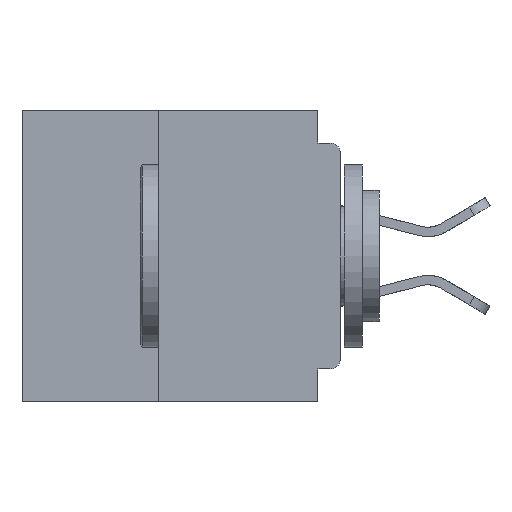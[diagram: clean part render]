
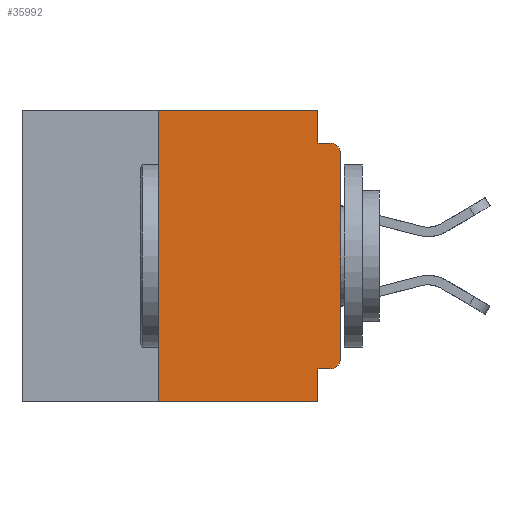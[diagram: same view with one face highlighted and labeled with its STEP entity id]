
A CAD part, left-side view. The second image highlights one B-rep face of the part: STEP entity #35992.
In plain terms, the highlighted planar face has unit normal (-1, 0, 0).
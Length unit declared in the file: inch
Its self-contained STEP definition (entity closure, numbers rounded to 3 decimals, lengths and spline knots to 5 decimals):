
#248 = VECTOR ( 'NONE', #33998, 39.37008 ) ;
#318 = VERTEX_POINT ( 'NONE', #36417 ) ;
#657 = CARTESIAN_POINT ( 'NONE',  ( 0., 0.031, -0.4 ) ) ;
#1243 = CARTESIAN_POINT ( 'NONE',  ( 0., 0.437, -0.4 ) ) ;
#1575 = CARTESIAN_POINT ( 'NONE',  ( 0., 0.015, -0.355 ) ) ;
#1850 = ORIENTED_EDGE ( 'NONE', *, *, #8075, .T. ) ;
#1880 = CARTESIAN_POINT ( 'NONE',  ( 0., 0.031, 0. ) ) ;
#3118 = VECTOR ( 'NONE', #18777, 39.37008 ) ;
#3287 = VECTOR ( 'NONE', #11905, 39.37008 ) ;
#3427 = VECTOR ( 'NONE', #29577, 39.37008 ) ;
#3503 = ORIENTED_EDGE ( 'NONE', *, *, #30465, .F. ) ;
#3931 = ORIENTED_EDGE ( 'NONE', *, *, #5375, .F. ) ;
#5300 = DIRECTION ( 'NONE',  ( 0., 0., -1. ) ) ;
#5311 = DIRECTION ( 'NONE',  ( -1., 0., 0. ) ) ;
#5351 = CARTESIAN_POINT ( 'NONE',  ( 0., 0.015, -0.06 ) ) ;
#5375 = EDGE_CURVE ( 'NONE', #17252, #19105, #22638, .T. ) ;
#5587 = EDGE_CURVE ( 'NONE', #14111, #20090, #9571, .T. ) ;
#5628 = AXIS2_PLACEMENT_3D ( 'NONE', #36807, #25675, #8404 ) ;
#6616 = DIRECTION ( 'NONE',  ( -1., 0., 0. ) ) ;
#6668 = VERTEX_POINT ( 'NONE', #29876 ) ;
#7271 = AXIS2_PLACEMENT_3D ( 'NONE', #5351, #5311, #5300 ) ;
#7435 = CARTESIAN_POINT ( 'NONE',  ( 0., 0.015, -0.045 ) ) ;
#7819 = DIRECTION ( 'NONE',  ( 0., -1., 0. ) ) ;
#8075 = EDGE_CURVE ( 'NONE', #25071, #19105, #21773, .T. ) ;
#8404 = DIRECTION ( 'NONE',  ( 0., 0., -1. ) ) ;
#8577 = CARTESIAN_POINT ( 'NONE',  ( 0., 0., -0.34 ) ) ;
#9366 = CARTESIAN_POINT ( 'NONE',  ( 0., 0., 0. ) ) ;
#9571 = LINE ( 'NONE', #26659, #26824 ) ;
#9645 = ORIENTED_EDGE ( 'NONE', *, *, #35458, .F. ) ;
#11087 = PLANE ( 'NONE',  #5628 ) ;
#11290 = LINE ( 'NONE', #17385, #18085 ) ;
#11348 = ORIENTED_EDGE ( 'NONE', *, *, #33555, .F. ) ;
#11905 = DIRECTION ( 'NONE',  ( 0., 0., -1. ) ) ;
#12288 = DIRECTION ( 'NONE',  ( 0., 0., 1. ) ) ;
#13571 = VECTOR ( 'NONE', #7819, 39.37008 ) ;
#13595 = CARTESIAN_POINT ( 'NONE',  ( 0., 0.437, 0. ) ) ;
#14111 = VERTEX_POINT ( 'NONE', #1575 ) ;
#15282 = ORIENTED_EDGE ( 'NONE', *, *, #31592, .T. ) ;
#15802 = VERTEX_POINT ( 'NONE', #26687 ) ;
#15805 = EDGE_CURVE ( 'NONE', #14111, #19342, #19909, .T. ) ;
#16256 = ORIENTED_EDGE ( 'NONE', *, *, #15805, .T. ) ;
#16298 = EDGE_CURVE ( 'NONE', #318, #15802, #11290, .T. ) ;
#16330 = CARTESIAN_POINT ( 'NONE',  ( 0., 0.031, -0.045 ) ) ;
#16380 = LINE ( 'NONE', #9366, #30622 ) ;
#17113 = ORIENTED_EDGE ( 'NONE', *, *, #37272, .T. ) ;
#17252 = VERTEX_POINT ( 'NONE', #16330 ) ;
#17385 = CARTESIAN_POINT ( 'NONE',  ( 0., 0.25, -0.4 ) ) ;
#18085 = VECTOR ( 'NONE', #23004, 39.37008 ) ;
#18777 = DIRECTION ( 'NONE',  ( 0., -1., 0. ) ) ;
#19105 = VERTEX_POINT ( 'NONE', #7435 ) ;
#19342 = VERTEX_POINT ( 'NONE', #8577 ) ;
#19470 = LINE ( 'NONE', #1243, #3118 ) ;
#19909 = CIRCLE ( 'NONE', #27265, 0.015 ) ;
#20090 = VERTEX_POINT ( 'NONE', #29636 ) ;
#20280 = CARTESIAN_POINT ( 'NONE',  ( 0., 0., -0.06 ) ) ;
#20659 = LINE ( 'NONE', #657, #3427 ) ;
#21188 = LINE ( 'NONE', #13595, #13571 ) ;
#21356 = ORIENTED_EDGE ( 'NONE', *, *, #5587, .F. ) ;
#21773 = CIRCLE ( 'NONE', #7271, 0.015 ) ;
#21817 = FACE_OUTER_BOUND ( 'NONE', #34241, .T. ) ;
#21901 = VERTEX_POINT ( 'NONE', #1880 ) ;
#22638 = LINE ( 'NONE', #34266, #248 ) ;
#23004 = DIRECTION ( 'NONE',  ( 0., 0., 1. ) ) ;
#23919 = CARTESIAN_POINT ( 'NONE',  ( 0., 0.015, -0.34 ) ) ;
#25071 = VERTEX_POINT ( 'NONE', #20280 ) ;
#25675 = DIRECTION ( 'NONE',  ( 1., 0., 0. ) ) ;
#26532 = DIRECTION ( 'NONE',  ( 0., 1., 0. ) ) ;
#26659 = CARTESIAN_POINT ( 'NONE',  ( 0., 0., -0.355 ) ) ;
#26687 = CARTESIAN_POINT ( 'NONE',  ( 0., 0.25, 0. ) ) ;
#26796 = DIRECTION ( 'NONE',  ( 0., 0., -1. ) ) ;
#26824 = VECTOR ( 'NONE', #26532, 39.37008 ) ;
#27265 = AXIS2_PLACEMENT_3D ( 'NONE', #23919, #6616, #26796 ) ;
#29052 = CARTESIAN_POINT ( 'NONE',  ( 0., 0.031, 0. ) ) ;
#29577 = DIRECTION ( 'NONE',  ( 0., 0., -1. ) ) ;
#29636 = CARTESIAN_POINT ( 'NONE',  ( 0., 0.031, -0.355 ) ) ;
#29876 = CARTESIAN_POINT ( 'NONE',  ( 0., 0.031, -0.4 ) ) ;
#30465 = EDGE_CURVE ( 'NONE', #15802, #21901, #21188, .T. ) ;
#30622 = VECTOR ( 'NONE', #12288, 39.37008 ) ;
#31592 = EDGE_CURVE ( 'NONE', #318, #6668, #19470, .T. ) ;
#32952 = LINE ( 'NONE', #29052, #3287 ) ;
#33064 = ORIENTED_EDGE ( 'NONE', *, *, #16298, .F. ) ;
#33555 = EDGE_CURVE ( 'NONE', #20090, #6668, #20659, .T. ) ;
#33998 = DIRECTION ( 'NONE',  ( 0., -1., 0. ) ) ;
#34241 = EDGE_LOOP ( 'NONE', ( #17113, #1850, #3931, #9645, #3503, #33064, #15282, #11348, #21356, #16256 ) ) ;
#34266 = CARTESIAN_POINT ( 'NONE',  ( 0., 0., -0.045 ) ) ;
#35458 = EDGE_CURVE ( 'NONE', #21901, #17252, #32952, .T. ) ;
#35992 = ADVANCED_FACE ( 'NONE', ( #21817 ), #11087, .F. ) ;
#36417 = CARTESIAN_POINT ( 'NONE',  ( 0., 0.25, -0.4 ) ) ;
#36807 = CARTESIAN_POINT ( 'NONE',  ( 0., 0.437, 0. ) ) ;
#37272 = EDGE_CURVE ( 'NONE', #19342, #25071, #16380, .T. ) ;
